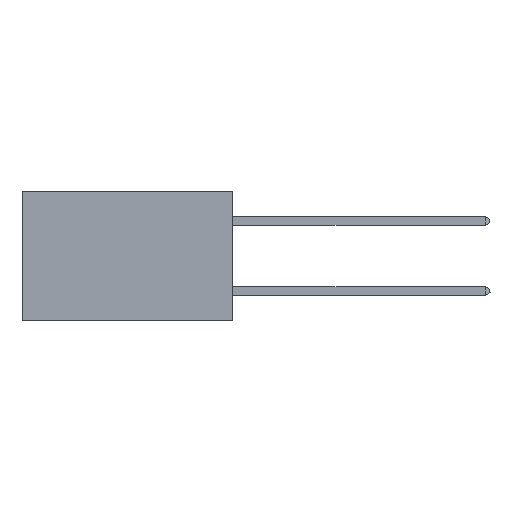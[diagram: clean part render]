
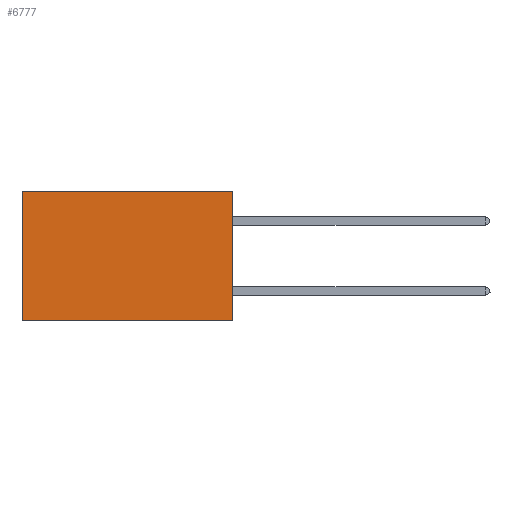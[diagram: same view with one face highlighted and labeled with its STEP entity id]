
A CAD part, left-side view. The second image highlights one B-rep face of the part: STEP entity #6777.
In plain terms, the highlighted planar face has unit normal (-1, 0, 0).
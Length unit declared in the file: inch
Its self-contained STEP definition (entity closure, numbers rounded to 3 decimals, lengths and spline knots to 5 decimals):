
#273 = DIRECTION ( 'NONE',  ( 0., 1., 0. ) ) ;
#402 = VECTOR ( 'NONE', #18029, 39.37008 ) ;
#1001 = LINE ( 'NONE', #14160, #23051 ) ;
#1092 = CARTESIAN_POINT ( 'NONE',  ( 0.2875, 0., 0. ) ) ;
#2840 = CARTESIAN_POINT ( 'NONE',  ( 0.2875, 0.6, -0.37 ) ) ;
#3239 = EDGE_LOOP ( 'NONE', ( #14376, #14069, #17581, #10359 ) ) ;
#3347 = CARTESIAN_POINT ( 'NONE',  ( 0.2875, 0., -0.37 ) ) ;
#3970 = EDGE_CURVE ( 'NONE', #12539, #22121, #1001, .T. ) ;
#4488 = VECTOR ( 'NONE', #8990, 39.37008 ) ;
#5152 = DIRECTION ( 'NONE',  ( 0., 0., -1. ) ) ;
#6060 = VECTOR ( 'NONE', #273, 39.37008 ) ;
#6185 = LINE ( 'NONE', #22206, #402 ) ;
#6777 = ADVANCED_FACE ( 'NONE', ( #10328 ), #16391, .F. ) ;
#6820 = EDGE_CURVE ( 'NONE', #22121, #16669, #9683, .T. ) ;
#8319 = DIRECTION ( 'NONE',  ( 0., 0., -1. ) ) ;
#8990 = DIRECTION ( 'NONE',  ( 0., 1., 0. ) ) ;
#9683 = LINE ( 'NONE', #3347, #4488 ) ;
#10328 = FACE_OUTER_BOUND ( 'NONE', #3239, .T. ) ;
#10359 = ORIENTED_EDGE ( 'NONE', *, *, #21117, .T. ) ;
#12502 = DIRECTION ( 'NONE',  ( 1., 0., 0. ) ) ;
#12539 = VERTEX_POINT ( 'NONE', #24047 ) ;
#14021 = LINE ( 'NONE', #14258, #6060 ) ;
#14069 = ORIENTED_EDGE ( 'NONE', *, *, #6820, .F. ) ;
#14160 = CARTESIAN_POINT ( 'NONE',  ( 0.2875, 0., 0. ) ) ;
#14258 = CARTESIAN_POINT ( 'NONE',  ( 0.2875, 0., 0. ) ) ;
#14376 = ORIENTED_EDGE ( 'NONE', *, *, #25227, .T. ) ;
#16391 = PLANE ( 'NONE',  #20363 ) ;
#16669 = VERTEX_POINT ( 'NONE', #2840 ) ;
#17581 = ORIENTED_EDGE ( 'NONE', *, *, #3970, .F. ) ;
#18029 = DIRECTION ( 'NONE',  ( 0., 0., -1. ) ) ;
#20029 = VERTEX_POINT ( 'NONE', #22060 ) ;
#20363 = AXIS2_PLACEMENT_3D ( 'NONE', #1092, #12502, #5152 ) ;
#21117 = EDGE_CURVE ( 'NONE', #12539, #20029, #14021, .T. ) ;
#21647 = CARTESIAN_POINT ( 'NONE',  ( 0.2875, 0., -0.37 ) ) ;
#22060 = CARTESIAN_POINT ( 'NONE',  ( 0.2875, 0.6, 0. ) ) ;
#22121 = VERTEX_POINT ( 'NONE', #21647 ) ;
#22206 = CARTESIAN_POINT ( 'NONE',  ( 0.2875, 0.6, 0. ) ) ;
#23051 = VECTOR ( 'NONE', #8319, 39.37008 ) ;
#24047 = CARTESIAN_POINT ( 'NONE',  ( 0.2875, 0., 0. ) ) ;
#25227 = EDGE_CURVE ( 'NONE', #20029, #16669, #6185, .T. ) ;
